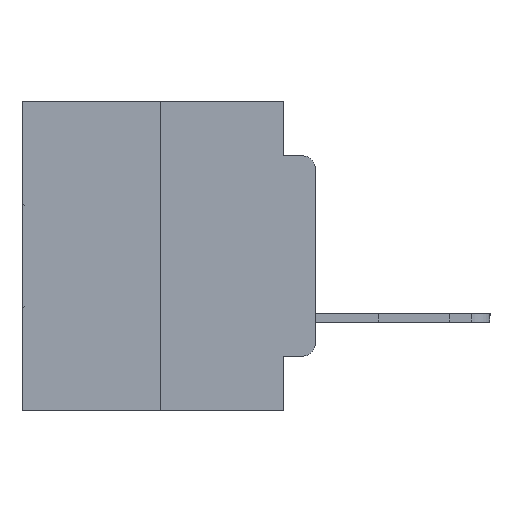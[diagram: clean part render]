
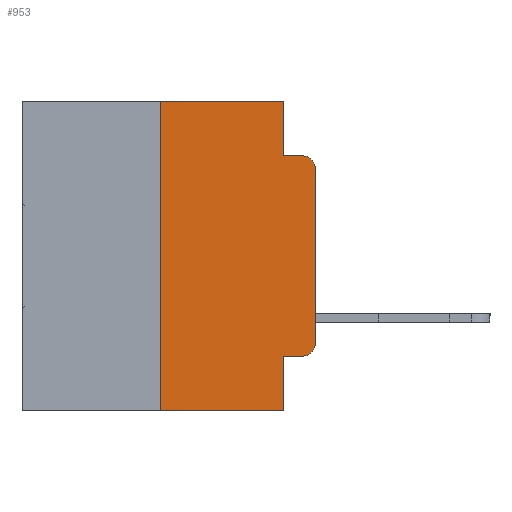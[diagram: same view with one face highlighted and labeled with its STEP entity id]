
A CAD part, left-side view. The second image highlights one B-rep face of the part: STEP entity #953.
In plain terms, the highlighted planar face has unit normal (-1, 0, 0).
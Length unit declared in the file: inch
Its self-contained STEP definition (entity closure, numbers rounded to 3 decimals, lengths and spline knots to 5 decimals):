
#189 = CARTESIAN_POINT ( 'NONE',  ( 0., 0.473, 0. ) ) ;
#663 = LINE ( 'NONE', #13697, #23923 ) ;
#724 = EDGE_CURVE ( 'NONE', #14252, #8037, #9001, .T. ) ;
#857 = ORIENTED_EDGE ( 'NONE', *, *, #12546, .T. ) ;
#953 = ADVANCED_FACE ( 'NONE', ( #10719 ), #27395, .F. ) ;
#1086 = EDGE_LOOP ( 'NONE', ( #857, #8411, #20271, #26158, #15760, #27579, #22354, #5213, #17170, #12572 ) ) ;
#1650 = CARTESIAN_POINT ( 'NONE',  ( 0., 0., 0. ) ) ;
#1942 = CARTESIAN_POINT ( 'NONE',  ( 0., 0.051, -0.0885 ) ) ;
#2208 = AXIS2_PLACEMENT_3D ( 'NONE', #27784, #14667, #26227 ) ;
#2556 = CIRCLE ( 'NONE', #12862, 0.02 ) ;
#3681 = DIRECTION ( 'NONE',  ( -1., 0., 0. ) ) ;
#4691 = CARTESIAN_POINT ( 'NONE',  ( 0., 0., -0.3915 ) ) ;
#4791 = VERTEX_POINT ( 'NONE', #21508 ) ;
#4954 = DIRECTION ( 'NONE',  ( 0., -1., 0. ) ) ;
#5213 = ORIENTED_EDGE ( 'NONE', *, *, #26929, .F. ) ;
#5326 = CARTESIAN_POINT ( 'NONE',  ( 0., 0.02, -0.0885 ) ) ;
#5641 = VERTEX_POINT ( 'NONE', #20030 ) ;
#6081 = DIRECTION ( 'NONE',  ( 0., 0., -1. ) ) ;
#7017 = LINE ( 'NONE', #24640, #24123 ) ;
#7541 = VECTOR ( 'NONE', #25215, 39.37008 ) ;
#7933 = CARTESIAN_POINT ( 'NONE',  ( 0., 0.051, -0.4115 ) ) ;
#8037 = VERTEX_POINT ( 'NONE', #1942 ) ;
#8354 = CARTESIAN_POINT ( 'NONE',  ( 0., 0.051, 0. ) ) ;
#8411 = ORIENTED_EDGE ( 'NONE', *, *, #27101, .T. ) ;
#8622 = VERTEX_POINT ( 'NONE', #11306 ) ;
#9001 = LINE ( 'NONE', #12124, #9695 ) ;
#9695 = VECTOR ( 'NONE', #6081, 39.37008 ) ;
#10318 = CARTESIAN_POINT ( 'NONE',  ( 0., 0.02, -0.3915 ) ) ;
#10719 = FACE_OUTER_BOUND ( 'NONE', #1086, .T. ) ;
#11306 = CARTESIAN_POINT ( 'NONE',  ( 0., 0., -0.1085 ) ) ;
#12124 = CARTESIAN_POINT ( 'NONE',  ( 0., 0.051, 0. ) ) ;
#12160 = LINE ( 'NONE', #7933, #18142 ) ;
#12545 = DIRECTION ( 'NONE',  ( 0., 0., -1. ) ) ;
#12546 = EDGE_CURVE ( 'NONE', #13989, #8622, #22474, .T. ) ;
#12572 = ORIENTED_EDGE ( 'NONE', *, *, #13664, .T. ) ;
#12835 = EDGE_CURVE ( 'NONE', #20410, #20984, #20718, .T. ) ;
#12862 = AXIS2_PLACEMENT_3D ( 'NONE', #17169, #3681, #19396 ) ;
#12998 = AXIS2_PLACEMENT_3D ( 'NONE', #10318, #25884, #12545 ) ;
#13664 = EDGE_CURVE ( 'NONE', #4791, #13989, #15440, .T. ) ;
#13697 = CARTESIAN_POINT ( 'NONE',  ( 0., 0.051, -0.0885 ) ) ;
#13951 = EDGE_CURVE ( 'NONE', #20410, #19598, #7017, .T. ) ;
#13989 = VERTEX_POINT ( 'NONE', #4691 ) ;
#14073 = VECTOR ( 'NONE', #4954, 39.37008 ) ;
#14252 = VERTEX_POINT ( 'NONE', #8354 ) ;
#14311 = CARTESIAN_POINT ( 'NONE',  ( 0., 0.051, 0. ) ) ;
#14667 = DIRECTION ( 'NONE',  ( 1., 0., 0. ) ) ;
#14738 = EDGE_CURVE ( 'NONE', #19598, #14252, #21615, .T. ) ;
#15010 = VECTOR ( 'NONE', #18339, 39.37008 ) ;
#15440 = CIRCLE ( 'NONE', #12998, 0.02 ) ;
#15760 = ORIENTED_EDGE ( 'NONE', *, *, #14738, .F. ) ;
#17169 = CARTESIAN_POINT ( 'NONE',  ( 0., 0.02, -0.1085 ) ) ;
#17170 = ORIENTED_EDGE ( 'NONE', *, *, #18469, .T. ) ;
#17279 = VECTOR ( 'NONE', #17450, 39.37008 ) ;
#17450 = DIRECTION ( 'NONE',  ( 0., 0., 1. ) ) ;
#18142 = VECTOR ( 'NONE', #23530, 39.37008 ) ;
#18339 = DIRECTION ( 'NONE',  ( 0., -1., 0. ) ) ;
#18469 = EDGE_CURVE ( 'NONE', #5641, #4791, #12160, .T. ) ;
#18740 = LINE ( 'NONE', #14311, #7541 ) ;
#18919 = CARTESIAN_POINT ( 'NONE',  ( 0., 0.25, 0. ) ) ;
#19396 = DIRECTION ( 'NONE',  ( 0., 0., -1. ) ) ;
#19598 = VERTEX_POINT ( 'NONE', #18919 ) ;
#20030 = CARTESIAN_POINT ( 'NONE',  ( 0., 0.051, -0.4115 ) ) ;
#20271 = ORIENTED_EDGE ( 'NONE', *, *, #27391, .F. ) ;
#20410 = VERTEX_POINT ( 'NONE', #28562 ) ;
#20613 = CARTESIAN_POINT ( 'NONE',  ( 0., 0.473, -0.5 ) ) ;
#20714 = VERTEX_POINT ( 'NONE', #5326 ) ;
#20718 = LINE ( 'NONE', #20613, #14073 ) ;
#20984 = VERTEX_POINT ( 'NONE', #26606 ) ;
#21508 = CARTESIAN_POINT ( 'NONE',  ( 0., 0.02, -0.4115 ) ) ;
#21615 = LINE ( 'NONE', #189, #15010 ) ;
#22354 = ORIENTED_EDGE ( 'NONE', *, *, #12835, .T. ) ;
#22474 = LINE ( 'NONE', #1650, #17279 ) ;
#23530 = DIRECTION ( 'NONE',  ( 0., -1., 0. ) ) ;
#23923 = VECTOR ( 'NONE', #24823, 39.37008 ) ;
#24123 = VECTOR ( 'NONE', #26862, 39.37008 ) ;
#24640 = CARTESIAN_POINT ( 'NONE',  ( 0., 0.25, 0. ) ) ;
#24823 = DIRECTION ( 'NONE',  ( 0., -1., 0. ) ) ;
#25215 = DIRECTION ( 'NONE',  ( 0., 0., -1. ) ) ;
#25884 = DIRECTION ( 'NONE',  ( -1., 0., 0. ) ) ;
#26158 = ORIENTED_EDGE ( 'NONE', *, *, #724, .F. ) ;
#26227 = DIRECTION ( 'NONE',  ( 0., 0., -1. ) ) ;
#26606 = CARTESIAN_POINT ( 'NONE',  ( 0., 0.051, -0.5 ) ) ;
#26862 = DIRECTION ( 'NONE',  ( 0., 0., 1. ) ) ;
#26929 = EDGE_CURVE ( 'NONE', #5641, #20984, #18740, .T. ) ;
#27101 = EDGE_CURVE ( 'NONE', #8622, #20714, #2556, .T. ) ;
#27391 = EDGE_CURVE ( 'NONE', #8037, #20714, #663, .T. ) ;
#27395 = PLANE ( 'NONE',  #2208 ) ;
#27579 = ORIENTED_EDGE ( 'NONE', *, *, #13951, .F. ) ;
#27784 = CARTESIAN_POINT ( 'NONE',  ( 0., 0.473, 0. ) ) ;
#28562 = CARTESIAN_POINT ( 'NONE',  ( 0., 0.25, -0.5 ) ) ;
